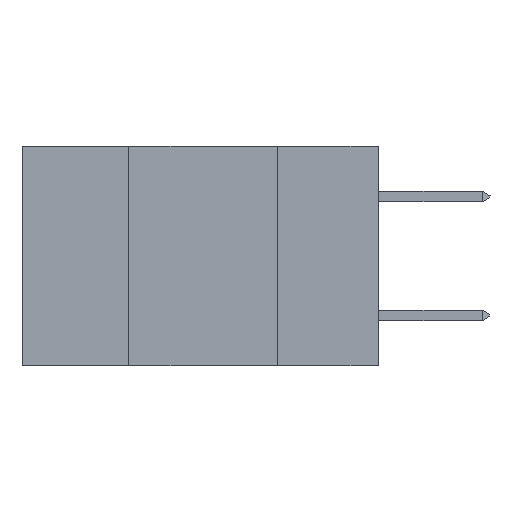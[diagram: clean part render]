
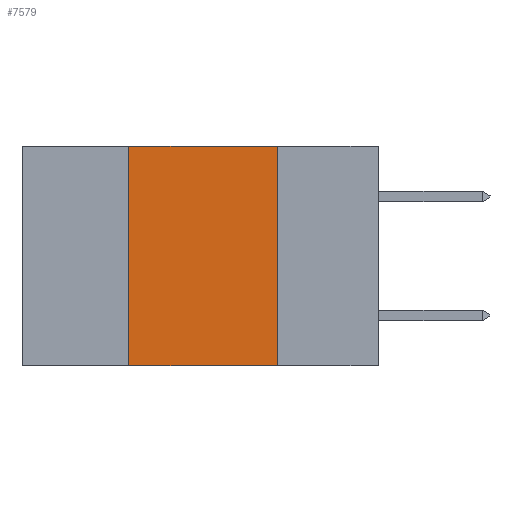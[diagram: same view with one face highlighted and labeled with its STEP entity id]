
A CAD part, left-side view. The second image highlights one B-rep face of the part: STEP entity #7579.
In plain terms, the highlighted planar face has unit normal (-1, 0, 0).
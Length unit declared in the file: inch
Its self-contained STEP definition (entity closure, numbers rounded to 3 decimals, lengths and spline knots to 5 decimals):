
#374 = ORIENTED_EDGE ( 'NONE', *, *, #11778, .T. ) ;
#772 = LINE ( 'NONE', #8696, #12782 ) ;
#1048 = ORIENTED_EDGE ( 'NONE', *, *, #11239, .F. ) ;
#1412 = DIRECTION ( 'NONE',  ( 0., -1., 0. ) ) ;
#2067 = EDGE_LOOP ( 'NONE', ( #11336, #1048, #2657, #374 ) ) ;
#2164 = AXIS2_PLACEMENT_3D ( 'NONE', #11986, #3043, #7028 ) ;
#2208 = VECTOR ( 'NONE', #2227, 39.37008 ) ;
#2227 = DIRECTION ( 'NONE',  ( 0., -1., 0. ) ) ;
#2657 = ORIENTED_EDGE ( 'NONE', *, *, #10129, .F. ) ;
#3043 = DIRECTION ( 'NONE',  ( 1., 0., 0. ) ) ;
#3187 = VERTEX_POINT ( 'NONE', #12377 ) ;
#3190 = LINE ( 'NONE', #10072, #2208 ) ;
#3421 = LINE ( 'NONE', #5383, #10357 ) ;
#4014 = FACE_OUTER_BOUND ( 'NONE', #2067, .T. ) ;
#5365 = DIRECTION ( 'NONE',  ( 0., 0., 1. ) ) ;
#5383 = CARTESIAN_POINT ( 'NONE',  ( 0., 0.6, -0.37 ) ) ;
#5442 = EDGE_CURVE ( 'NONE', #12376, #3187, #772, .T. ) ;
#5720 = VERTEX_POINT ( 'NONE', #7174 ) ;
#6551 = CARTESIAN_POINT ( 'NONE',  ( 0., 0.17, 0. ) ) ;
#7028 = DIRECTION ( 'NONE',  ( 0., 0., -1. ) ) ;
#7174 = CARTESIAN_POINT ( 'NONE',  ( 0., 0.42, -0.37 ) ) ;
#7579 = ADVANCED_FACE ( 'NONE', ( #4014 ), #8016, .F. ) ;
#7925 = CARTESIAN_POINT ( 'NONE',  ( 0., 0.42, 0. ) ) ;
#8016 = PLANE ( 'NONE',  #2164 ) ;
#8696 = CARTESIAN_POINT ( 'NONE',  ( 0., 0.17, -0.37 ) ) ;
#8872 = VECTOR ( 'NONE', #5365, 39.37008 ) ;
#10072 = CARTESIAN_POINT ( 'NONE',  ( 0., 0.6, 0. ) ) ;
#10129 = EDGE_CURVE ( 'NONE', #5720, #12111, #10365, .T. ) ;
#10357 = VECTOR ( 'NONE', #1412, 39.37008 ) ;
#10365 = LINE ( 'NONE', #11311, #8872 ) ;
#11239 = EDGE_CURVE ( 'NONE', #12111, #12376, #3190, .T. ) ;
#11311 = CARTESIAN_POINT ( 'NONE',  ( 0., 0.42, -0.37 ) ) ;
#11336 = ORIENTED_EDGE ( 'NONE', *, *, #5442, .F. ) ;
#11778 = EDGE_CURVE ( 'NONE', #5720, #3187, #3421, .T. ) ;
#11986 = CARTESIAN_POINT ( 'NONE',  ( 0., 0.6, 0. ) ) ;
#12111 = VERTEX_POINT ( 'NONE', #7925 ) ;
#12376 = VERTEX_POINT ( 'NONE', #6551 ) ;
#12377 = CARTESIAN_POINT ( 'NONE',  ( 0., 0.17, -0.37 ) ) ;
#12719 = DIRECTION ( 'NONE',  ( 0., 0., -1. ) ) ;
#12782 = VECTOR ( 'NONE', #12719, 39.37008 ) ;
